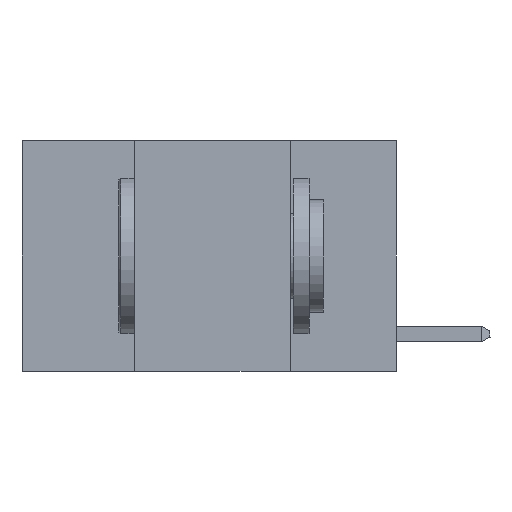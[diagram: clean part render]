
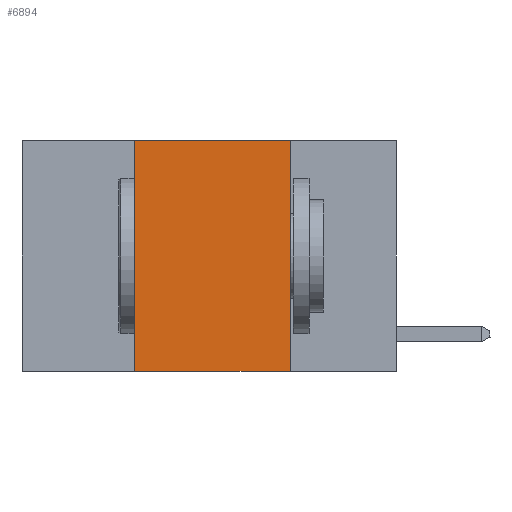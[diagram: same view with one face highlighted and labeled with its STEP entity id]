
A CAD part, left-side view. The second image highlights one B-rep face of the part: STEP entity #6894.
In plain terms, the highlighted planar face has unit normal (-1, 0, 0).
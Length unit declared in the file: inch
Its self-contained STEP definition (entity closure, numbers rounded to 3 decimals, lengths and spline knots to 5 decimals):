
#258 = CARTESIAN_POINT ( 'NONE',  ( 0., 0.6, 0. ) ) ;
#297 = VERTEX_POINT ( 'NONE', #8999 ) ;
#330 = DIRECTION ( 'NONE',  ( 1., 0., 0. ) ) ;
#432 = CARTESIAN_POINT ( 'NONE',  ( 0., 0.42, -0.37 ) ) ;
#1970 = LINE ( 'NONE', #12901, #8880 ) ;
#2152 = CARTESIAN_POINT ( 'NONE',  ( 0., 0.17, -0.37 ) ) ;
#2233 = ORIENTED_EDGE ( 'NONE', *, *, #5271, .F. ) ;
#2407 = VECTOR ( 'NONE', #12397, 39.37008 ) ;
#3015 = VECTOR ( 'NONE', #11625, 39.37008 ) ;
#3242 = LINE ( 'NONE', #11913, #12310 ) ;
#4684 = DIRECTION ( 'NONE',  ( 0., 0., -1. ) ) ;
#4730 = CARTESIAN_POINT ( 'NONE',  ( 0., 0.42, 0. ) ) ;
#4759 = EDGE_CURVE ( 'NONE', #5059, #8792, #1970, .T. ) ;
#4827 = ORIENTED_EDGE ( 'NONE', *, *, #9422, .F. ) ;
#4902 = ORIENTED_EDGE ( 'NONE', *, *, #4759, .T. ) ;
#5059 = VERTEX_POINT ( 'NONE', #432 ) ;
#5271 = EDGE_CURVE ( 'NONE', #5059, #6046, #3242, .T. ) ;
#5321 = AXIS2_PLACEMENT_3D ( 'NONE', #258, #330, #4684 ) ;
#5988 = CARTESIAN_POINT ( 'NONE',  ( 0., 0.6, 0. ) ) ;
#6046 = VERTEX_POINT ( 'NONE', #4730 ) ;
#6530 = DIRECTION ( 'NONE',  ( 0., 0., 1. ) ) ;
#6802 = PLANE ( 'NONE',  #5321 ) ;
#6894 = ADVANCED_FACE ( 'NONE', ( #10152 ), #6802, .F. ) ;
#8400 = EDGE_CURVE ( 'NONE', #6046, #297, #9123, .T. ) ;
#8792 = VERTEX_POINT ( 'NONE', #2152 ) ;
#8880 = VECTOR ( 'NONE', #9749, 39.37008 ) ;
#8999 = CARTESIAN_POINT ( 'NONE',  ( 0., 0.17, 0. ) ) ;
#9123 = LINE ( 'NONE', #5988, #2407 ) ;
#9422 = EDGE_CURVE ( 'NONE', #297, #8792, #9579, .T. ) ;
#9579 = LINE ( 'NONE', #11750, #3015 ) ;
#9749 = DIRECTION ( 'NONE',  ( 0., -1., 0. ) ) ;
#10139 = EDGE_LOOP ( 'NONE', ( #4827, #13009, #2233, #4902 ) ) ;
#10152 = FACE_OUTER_BOUND ( 'NONE', #10139, .T. ) ;
#11625 = DIRECTION ( 'NONE',  ( 0., 0., -1. ) ) ;
#11750 = CARTESIAN_POINT ( 'NONE',  ( 0., 0.17, 0. ) ) ;
#11913 = CARTESIAN_POINT ( 'NONE',  ( 0., 0.42, 0. ) ) ;
#12310 = VECTOR ( 'NONE', #6530, 39.37008 ) ;
#12397 = DIRECTION ( 'NONE',  ( 0., -1., 0. ) ) ;
#12901 = CARTESIAN_POINT ( 'NONE',  ( 0., 0.6, -0.37 ) ) ;
#13009 = ORIENTED_EDGE ( 'NONE', *, *, #8400, .F. ) ;
